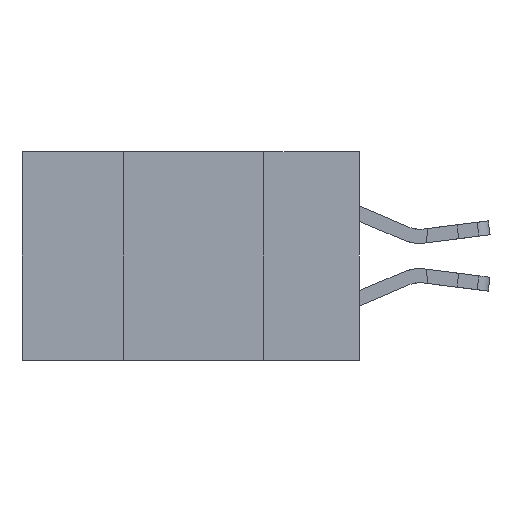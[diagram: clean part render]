
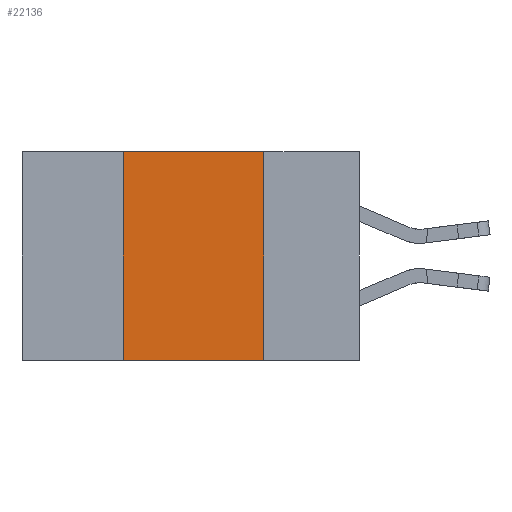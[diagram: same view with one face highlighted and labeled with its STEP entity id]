
A CAD part, left-side view. The second image highlights one B-rep face of the part: STEP entity #22136.
In plain terms, the highlighted planar face has unit normal (-1, 0, 0).
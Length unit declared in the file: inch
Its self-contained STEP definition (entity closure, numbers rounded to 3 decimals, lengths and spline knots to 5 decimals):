
#2446 = ORIENTED_EDGE ( 'NONE', *, *, #21960, .T. ) ;
#2612 = ORIENTED_EDGE ( 'NONE', *, *, #3865, .F. ) ;
#3865 = EDGE_CURVE ( 'NONE', #13799, #19386, #11106, .T. ) ;
#4049 = CARTESIAN_POINT ( 'NONE',  ( 0., 0.6, -0.37 ) ) ;
#4241 = CARTESIAN_POINT ( 'NONE',  ( 0., 0.42, 0. ) ) ;
#4401 = PLANE ( 'NONE',  #16473 ) ;
#4870 = CARTESIAN_POINT ( 'NONE',  ( 0., 0.42, 0. ) ) ;
#5046 = VERTEX_POINT ( 'NONE', #18225 ) ;
#5058 = CARTESIAN_POINT ( 'NONE',  ( 0., 0.42, -0.37 ) ) ;
#5774 = VECTOR ( 'NONE', #13714, 39.37008 ) ;
#6035 = CARTESIAN_POINT ( 'NONE',  ( 0., 0.6, 0. ) ) ;
#6320 = LINE ( 'NONE', #4049, #16090 ) ;
#6631 = CARTESIAN_POINT ( 'NONE',  ( 0., 0.17, 0. ) ) ;
#7262 = ORIENTED_EDGE ( 'NONE', *, *, #17512, .F. ) ;
#9414 = EDGE_CURVE ( 'NONE', #15296, #5046, #21169, .T. ) ;
#10933 = VECTOR ( 'NONE', #13458, 39.37008 ) ;
#11106 = LINE ( 'NONE', #4870, #5774 ) ;
#11673 = VECTOR ( 'NONE', #16737, 39.37008 ) ;
#13215 = ORIENTED_EDGE ( 'NONE', *, *, #9414, .F. ) ;
#13458 = DIRECTION ( 'NONE',  ( 0., 0., -1. ) ) ;
#13714 = DIRECTION ( 'NONE',  ( 0., 0., 1. ) ) ;
#13799 = VERTEX_POINT ( 'NONE', #5058 ) ;
#13861 = CARTESIAN_POINT ( 'NONE',  ( 0., 0.6, 0. ) ) ;
#14846 = DIRECTION ( 'NONE',  ( 0., -1., 0. ) ) ;
#14952 = CARTESIAN_POINT ( 'NONE',  ( 0., 0.17, 0. ) ) ;
#15296 = VERTEX_POINT ( 'NONE', #14952 ) ;
#15528 = FACE_OUTER_BOUND ( 'NONE', #20668, .T. ) ;
#16090 = VECTOR ( 'NONE', #14846, 39.37008 ) ;
#16473 = AXIS2_PLACEMENT_3D ( 'NONE', #13861, #20139, #19326 ) ;
#16737 = DIRECTION ( 'NONE',  ( 0., -1., 0. ) ) ;
#17512 = EDGE_CURVE ( 'NONE', #19386, #15296, #17764, .T. ) ;
#17764 = LINE ( 'NONE', #6035, #11673 ) ;
#18225 = CARTESIAN_POINT ( 'NONE',  ( 0., 0.17, -0.37 ) ) ;
#19326 = DIRECTION ( 'NONE',  ( 0., 0., -1. ) ) ;
#19386 = VERTEX_POINT ( 'NONE', #4241 ) ;
#20139 = DIRECTION ( 'NONE',  ( 1., 0., 0. ) ) ;
#20668 = EDGE_LOOP ( 'NONE', ( #13215, #7262, #2612, #2446 ) ) ;
#21169 = LINE ( 'NONE', #6631, #10933 ) ;
#21960 = EDGE_CURVE ( 'NONE', #13799, #5046, #6320, .T. ) ;
#22136 = ADVANCED_FACE ( 'NONE', ( #15528 ), #4401, .F. ) ;
